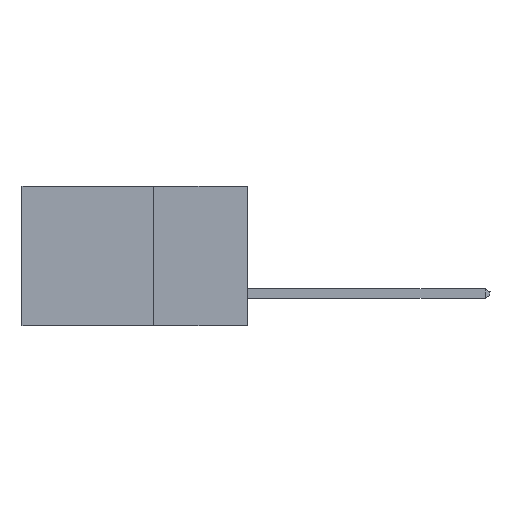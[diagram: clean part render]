
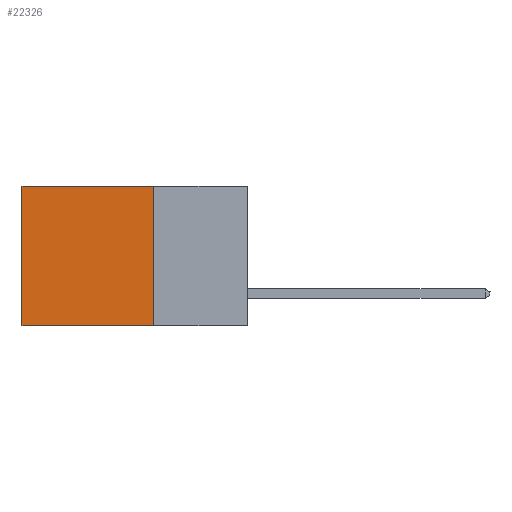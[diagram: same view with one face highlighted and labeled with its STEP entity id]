
A CAD part, left-side view. The second image highlights one B-rep face of the part: STEP entity #22326.
In plain terms, the highlighted planar face has unit normal (-1, 0, 0).
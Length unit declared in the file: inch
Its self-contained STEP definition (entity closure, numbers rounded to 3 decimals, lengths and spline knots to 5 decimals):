
#126 = DIRECTION ( 'NONE',  ( 0., 0., -1. ) ) ;
#1132 = VECTOR ( 'NONE', #6134, 39.37008 ) ;
#1167 = CARTESIAN_POINT ( 'NONE',  ( 0.2615, 0.25, 0. ) ) ;
#2775 = CARTESIAN_POINT ( 'NONE',  ( 0.2615, 0.25, -0.37 ) ) ;
#2966 = CARTESIAN_POINT ( 'NONE',  ( 0.2615, 0.25, 0. ) ) ;
#3002 = LINE ( 'NONE', #1167, #1132 ) ;
#3783 = CARTESIAN_POINT ( 'NONE',  ( 0.2615, 0.6, -0.37 ) ) ;
#6134 = DIRECTION ( 'NONE',  ( 0., 1., 0. ) ) ;
#6603 = EDGE_CURVE ( 'NONE', #10469, #17795, #8234, .T. ) ;
#6809 = DIRECTION ( 'NONE',  ( 0., 0., -1. ) ) ;
#8194 = VECTOR ( 'NONE', #16543, 39.37008 ) ;
#8234 = LINE ( 'NONE', #2775, #15385 ) ;
#8791 = CARTESIAN_POINT ( 'NONE',  ( 0.2615, 0.25, -0.37 ) ) ;
#10399 = FACE_OUTER_BOUND ( 'NONE', #13905, .T. ) ;
#10469 = VERTEX_POINT ( 'NONE', #14696 ) ;
#10513 = CARTESIAN_POINT ( 'NONE',  ( 0.2615, 0.25, -0.37 ) ) ;
#11271 = AXIS2_PLACEMENT_3D ( 'NONE', #10513, #15807, #6809 ) ;
#11663 = CARTESIAN_POINT ( 'NONE',  ( 0.2615, 0.6, 0. ) ) ;
#13905 = EDGE_LOOP ( 'NONE', ( #21456, #17995, #20348, #15373 ) ) ;
#14663 = EDGE_CURVE ( 'NONE', #21426, #16287, #3002, .T. ) ;
#14696 = CARTESIAN_POINT ( 'NONE',  ( 0.2615, 0.25, -0.37 ) ) ;
#14931 = CARTESIAN_POINT ( 'NONE',  ( 0.2615, 0.6, -0.37 ) ) ;
#15373 = ORIENTED_EDGE ( 'NONE', *, *, #14663, .T. ) ;
#15385 = VECTOR ( 'NONE', #20788, 39.37008 ) ;
#15773 = EDGE_CURVE ( 'NONE', #16287, #17795, #16659, .T. ) ;
#15807 = DIRECTION ( 'NONE',  ( 1., 0., 0. ) ) ;
#15951 = LINE ( 'NONE', #8791, #21822 ) ;
#16117 = EDGE_CURVE ( 'NONE', #21426, #10469, #15951, .T. ) ;
#16287 = VERTEX_POINT ( 'NONE', #11663 ) ;
#16543 = DIRECTION ( 'NONE',  ( 0., 0., -1. ) ) ;
#16659 = LINE ( 'NONE', #14931, #8194 ) ;
#17552 = PLANE ( 'NONE',  #11271 ) ;
#17795 = VERTEX_POINT ( 'NONE', #3783 ) ;
#17995 = ORIENTED_EDGE ( 'NONE', *, *, #6603, .F. ) ;
#20348 = ORIENTED_EDGE ( 'NONE', *, *, #16117, .F. ) ;
#20788 = DIRECTION ( 'NONE',  ( 0., 1., 0. ) ) ;
#21426 = VERTEX_POINT ( 'NONE', #2966 ) ;
#21456 = ORIENTED_EDGE ( 'NONE', *, *, #15773, .T. ) ;
#21822 = VECTOR ( 'NONE', #126, 39.37008 ) ;
#22326 = ADVANCED_FACE ( 'NONE', ( #10399 ), #17552, .F. ) ;
